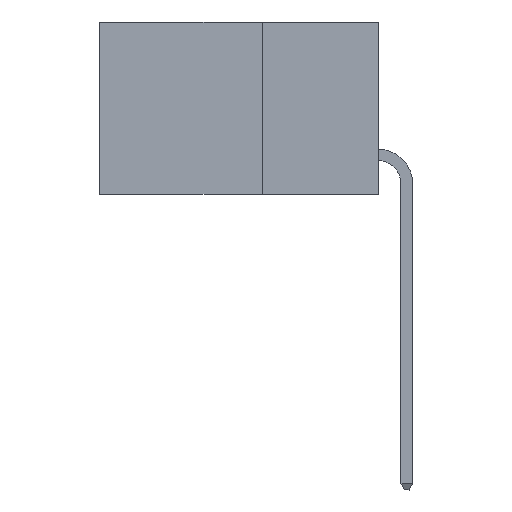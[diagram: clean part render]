
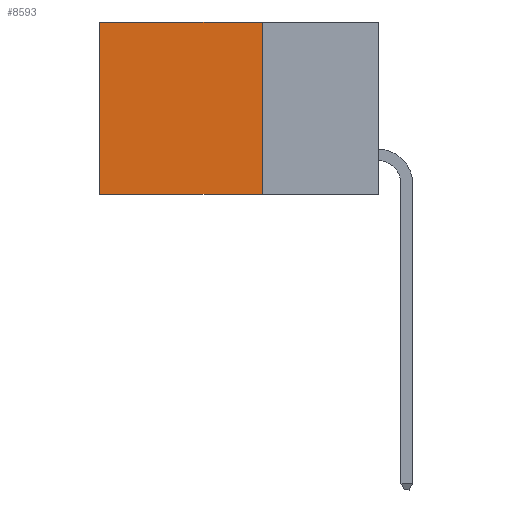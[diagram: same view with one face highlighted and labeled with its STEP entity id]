
A CAD part, left-side view. The second image highlights one B-rep face of the part: STEP entity #8593.
In plain terms, the highlighted planar face has unit normal (-1, 0, 0).
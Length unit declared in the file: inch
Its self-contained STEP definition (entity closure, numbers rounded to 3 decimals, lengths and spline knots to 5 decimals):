
#132 = CARTESIAN_POINT ( 'NONE',  ( 0.298, 0.6, 0. ) ) ;
#842 = DIRECTION ( 'NONE',  ( 0., 1., 0. ) ) ;
#1582 = CARTESIAN_POINT ( 'NONE',  ( 0.298, 0.25, 0. ) ) ;
#1688 = DIRECTION ( 'NONE',  ( 0., 0., -1. ) ) ;
#1957 = DIRECTION ( 'NONE',  ( 0., 1., 0. ) ) ;
#2517 = EDGE_CURVE ( 'NONE', #10552, #8589, #10182, .T. ) ;
#2753 = CARTESIAN_POINT ( 'NONE',  ( 0.298, 0.25, 0. ) ) ;
#2829 = ORIENTED_EDGE ( 'NONE', *, *, #2517, .F. ) ;
#3142 = LINE ( 'NONE', #14455, #10645 ) ;
#3401 = CARTESIAN_POINT ( 'NONE',  ( 0.298, 0.6, 0. ) ) ;
#3528 = ORIENTED_EDGE ( 'NONE', *, *, #5130, .F. ) ;
#3724 = CARTESIAN_POINT ( 'NONE',  ( 0.298, 0.6, -0.37 ) ) ;
#4021 = VERTEX_POINT ( 'NONE', #3724 ) ;
#4303 = VECTOR ( 'NONE', #12565, 39.37008 ) ;
#4621 = DIRECTION ( 'NONE',  ( 1., 0., 0. ) ) ;
#5130 = EDGE_CURVE ( 'NONE', #8589, #4021, #12982, .T. ) ;
#5720 = CARTESIAN_POINT ( 'NONE',  ( 0.298, 0.25, 0. ) ) ;
#6134 = ORIENTED_EDGE ( 'NONE', *, *, #7813, .T. ) ;
#6520 = VERTEX_POINT ( 'NONE', #132 ) ;
#7666 = ORIENTED_EDGE ( 'NONE', *, *, #10262, .T. ) ;
#7813 = EDGE_CURVE ( 'NONE', #6520, #4021, #10360, .T. ) ;
#8589 = VERTEX_POINT ( 'NONE', #11355 ) ;
#8593 = ADVANCED_FACE ( 'NONE', ( #10862 ), #10335, .F. ) ;
#9657 = VECTOR ( 'NONE', #1688, 39.37008 ) ;
#10182 = LINE ( 'NONE', #2753, #9657 ) ;
#10259 = AXIS2_PLACEMENT_3D ( 'NONE', #5720, #4621, #13647 ) ;
#10262 = EDGE_CURVE ( 'NONE', #10552, #6520, #3142, .T. ) ;
#10335 = PLANE ( 'NONE',  #10259 ) ;
#10360 = LINE ( 'NONE', #3401, #4303 ) ;
#10552 = VERTEX_POINT ( 'NONE', #1582 ) ;
#10645 = VECTOR ( 'NONE', #1957, 39.37008 ) ;
#10862 = FACE_OUTER_BOUND ( 'NONE', #11941, .T. ) ;
#11355 = CARTESIAN_POINT ( 'NONE',  ( 0.298, 0.25, -0.37 ) ) ;
#11941 = EDGE_LOOP ( 'NONE', ( #6134, #3528, #2829, #7666 ) ) ;
#12565 = DIRECTION ( 'NONE',  ( 0., 0., -1. ) ) ;
#12791 = VECTOR ( 'NONE', #842, 39.37008 ) ;
#12982 = LINE ( 'NONE', #14511, #12791 ) ;
#13647 = DIRECTION ( 'NONE',  ( 0., 0., -1. ) ) ;
#14455 = CARTESIAN_POINT ( 'NONE',  ( 0.298, 0.25, 0. ) ) ;
#14511 = CARTESIAN_POINT ( 'NONE',  ( 0.298, 0.25, -0.37 ) ) ;
